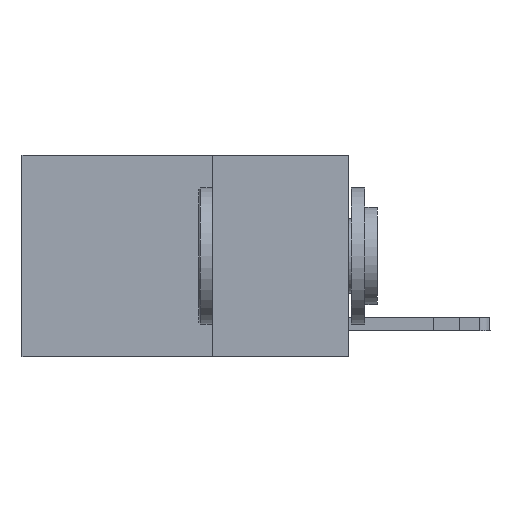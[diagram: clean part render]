
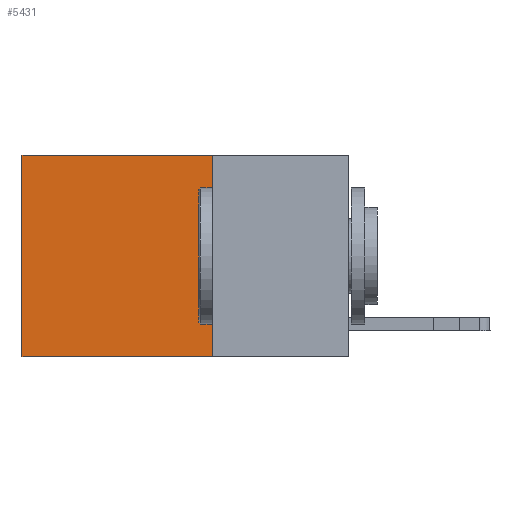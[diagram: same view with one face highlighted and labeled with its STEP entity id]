
A CAD part, left-side view. The second image highlights one B-rep face of the part: STEP entity #5431.
In plain terms, the highlighted planar face has unit normal (-1, 0, 0).
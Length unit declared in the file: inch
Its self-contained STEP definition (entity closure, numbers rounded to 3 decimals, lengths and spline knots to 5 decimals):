
#128 = CARTESIAN_POINT ( 'NONE',  ( 0.2625, 0.6, -0.37 ) ) ;
#1128 = VERTEX_POINT ( 'NONE', #3836 ) ;
#1217 = EDGE_LOOP ( 'NONE', ( #21547, #18420, #4850, #22550 ) ) ;
#2493 = CARTESIAN_POINT ( 'NONE',  ( 0.2625, 0.25, 0. ) ) ;
#2564 = DIRECTION ( 'NONE',  ( 0., 0., -1. ) ) ;
#3741 = LINE ( 'NONE', #9231, #7096 ) ;
#3802 = CARTESIAN_POINT ( 'NONE',  ( 0.2625, 0.25, 0. ) ) ;
#3836 = CARTESIAN_POINT ( 'NONE',  ( 0.2625, 0.25, -0.37 ) ) ;
#4533 = CARTESIAN_POINT ( 'NONE',  ( 0.2625, 0.25, 0. ) ) ;
#4755 = AXIS2_PLACEMENT_3D ( 'NONE', #2493, #6156, #13215 ) ;
#4850 = ORIENTED_EDGE ( 'NONE', *, *, #22843, .F. ) ;
#5384 = LINE ( 'NONE', #12546, #20457 ) ;
#5431 = ADVANCED_FACE ( 'NONE', ( #22215 ), #6034, .F. ) ;
#6034 = PLANE ( 'NONE',  #4755 ) ;
#6156 = DIRECTION ( 'NONE',  ( 1., 0., 0. ) ) ;
#6171 = EDGE_CURVE ( 'NONE', #1128, #21293, #5384, .T. ) ;
#7096 = VECTOR ( 'NONE', #18525, 39.37008 ) ;
#7101 = VERTEX_POINT ( 'NONE', #3802 ) ;
#7468 = VECTOR ( 'NONE', #2564, 39.37008 ) ;
#9231 = CARTESIAN_POINT ( 'NONE',  ( 0.2625, 0.6, 0. ) ) ;
#11698 = DIRECTION ( 'NONE',  ( 0., 1., 0. ) ) ;
#11959 = VECTOR ( 'NONE', #11698, 39.37008 ) ;
#12546 = CARTESIAN_POINT ( 'NONE',  ( 0.2625, 0.25, -0.37 ) ) ;
#13215 = DIRECTION ( 'NONE',  ( 0., 0., -1. ) ) ;
#13734 = LINE ( 'NONE', #4533, #11959 ) ;
#17018 = CARTESIAN_POINT ( 'NONE',  ( 0.2625, 0.25, 0. ) ) ;
#18420 = ORIENTED_EDGE ( 'NONE', *, *, #6171, .F. ) ;
#18525 = DIRECTION ( 'NONE',  ( 0., 0., -1. ) ) ;
#19668 = DIRECTION ( 'NONE',  ( 0., 1., 0. ) ) ;
#20457 = VECTOR ( 'NONE', #19668, 39.37008 ) ;
#20743 = LINE ( 'NONE', #17018, #7468 ) ;
#20777 = VERTEX_POINT ( 'NONE', #23038 ) ;
#21293 = VERTEX_POINT ( 'NONE', #128 ) ;
#21547 = ORIENTED_EDGE ( 'NONE', *, *, #23009, .T. ) ;
#22056 = EDGE_CURVE ( 'NONE', #7101, #20777, #13734, .T. ) ;
#22215 = FACE_OUTER_BOUND ( 'NONE', #1217, .T. ) ;
#22550 = ORIENTED_EDGE ( 'NONE', *, *, #22056, .T. ) ;
#22843 = EDGE_CURVE ( 'NONE', #7101, #1128, #20743, .T. ) ;
#23009 = EDGE_CURVE ( 'NONE', #20777, #21293, #3741, .T. ) ;
#23038 = CARTESIAN_POINT ( 'NONE',  ( 0.2625, 0.6, 0. ) ) ;
